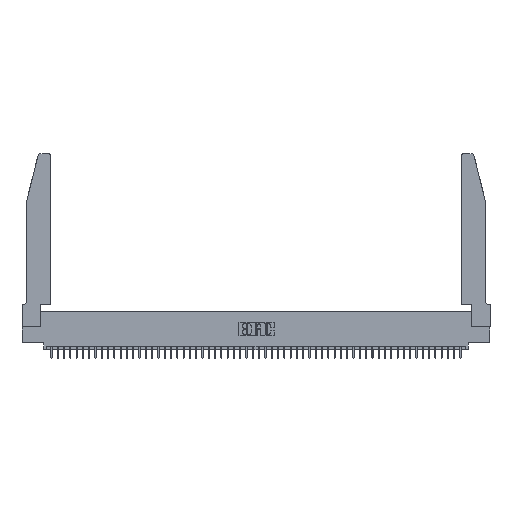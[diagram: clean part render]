
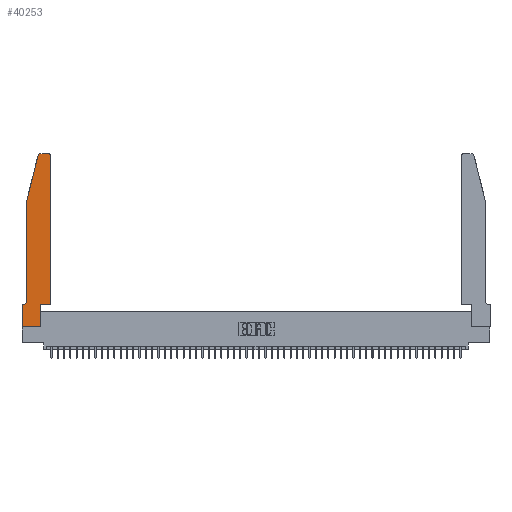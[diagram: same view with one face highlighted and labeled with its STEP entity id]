
A CAD part, top view. The second image highlights one B-rep face of the part: STEP entity #40253.
In plain terms, the highlighted planar face has unit normal (0, 0, 1).
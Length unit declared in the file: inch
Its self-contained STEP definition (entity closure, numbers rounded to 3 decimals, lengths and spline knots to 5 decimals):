
#1168 = CARTESIAN_POINT ( 'NONE',  ( 0.4505, 0.35, 0.37 ) ) ;
#1731 = LINE ( 'NONE', #50038, #8873 ) ;
#2999 = ORIENTED_EDGE ( 'NONE', *, *, #24528, .T. ) ;
#3394 = LINE ( 'NONE', #49758, #8717 ) ;
#3567 = DIRECTION ( 'NONE',  ( -0.239, -0.971, 0. ) ) ;
#3922 = VECTOR ( 'NONE', #53057, 39.37008 ) ;
#4249 = CARTESIAN_POINT ( 'NONE',  ( 0.0055, 0.35, 0.37 ) ) ;
#4438 = CARTESIAN_POINT ( 'NONE',  ( 0.0755, 0.35, 0.37 ) ) ;
#4554 = ORIENTED_EDGE ( 'NONE', *, *, #28800, .T. ) ;
#4902 = CARTESIAN_POINT ( 'NONE',  ( 0.2865, 0.35, 0.37 ) ) ;
#5096 = VECTOR ( 'NONE', #22157, 39.37008 ) ;
#5981 = ORIENTED_EDGE ( 'NONE', *, *, #35964, .T. ) ;
#6367 = ORIENTED_EDGE ( 'NONE', *, *, #37908, .T. ) ;
#6653 = DIRECTION ( 'NONE',  ( 0., -1., 0. ) ) ;
#7056 = CARTESIAN_POINT ( 'NONE',  ( 0.284, 2.75, 0.37 ) ) ;
#7441 = LINE ( 'NONE', #32641, #24389 ) ;
#7539 = CARTESIAN_POINT ( 'NONE',  ( 0.4505, 0.35, 0.37 ) ) ;
#7691 = DIRECTION ( 'NONE',  ( 1., 0., 0. ) ) ;
#7770 = ORIENTED_EDGE ( 'NONE', *, *, #14251, .T. ) ;
#8327 = DIRECTION ( 'NONE',  ( 0., 1., 0. ) ) ;
#8717 = VECTOR ( 'NONE', #20447, 39.37008 ) ;
#8873 = VECTOR ( 'NONE', #37860, 39.37008 ) ;
#9023 = LINE ( 'NONE', #4438, #3922 ) ;
#9691 = LINE ( 'NONE', #26239, #5096 ) ;
#9996 = CIRCLE ( 'NONE', #29907, 0.03 ) ;
#11538 = CARTESIAN_POINT ( 'NONE',  ( 0.4205, 2.72, 0.37 ) ) ;
#12077 = DIRECTION ( 'NONE',  ( 1., 0., 0. ) ) ;
#12919 = ORIENTED_EDGE ( 'NONE', *, *, #52742, .T. ) ;
#13733 = PLANE ( 'NONE',  #42702 ) ;
#13891 = ORIENTED_EDGE ( 'NONE', *, *, #16941, .T. ) ;
#14251 = EDGE_CURVE ( 'NONE', #24270, #21484, #44726, .T. ) ;
#14649 = DIRECTION ( 'NONE',  ( -1., 0., 0. ) ) ;
#16587 = CARTESIAN_POINT ( 'NONE',  ( 0.2865, 0., 0.37 ) ) ;
#16941 = EDGE_CURVE ( 'NONE', #29308, #30890, #9691, .T. ) ;
#19548 = CARTESIAN_POINT ( 'NONE',  ( 0.0755, 2., 0.37 ) ) ;
#19791 = VECTOR ( 'NONE', #32845, 39.37008 ) ;
#20447 = DIRECTION ( 'NONE',  ( 0., -1., 0. ) ) ;
#20902 = ORIENTED_EDGE ( 'NONE', *, *, #30260, .T. ) ;
#21484 = VERTEX_POINT ( 'NONE', #38367 ) ;
#22006 = DIRECTION ( 'NONE',  ( 1., 0., 0. ) ) ;
#22157 = DIRECTION ( 'NONE',  ( 0., 1., 0. ) ) ;
#22595 = CARTESIAN_POINT ( 'NONE',  ( 0.0755, 0.42, 0.37 ) ) ;
#22673 = DIRECTION ( 'NONE',  ( 0., 0., 1. ) ) ;
#22874 = CIRCLE ( 'NONE', #46230, 0.03 ) ;
#23353 = CARTESIAN_POINT ( 'NONE',  ( 0., 0.35, 0.37 ) ) ;
#23642 = LINE ( 'NONE', #19548, #27076 ) ;
#24270 = VERTEX_POINT ( 'NONE', #1168 ) ;
#24389 = VECTOR ( 'NONE', #7691, 39.37008 ) ;
#24528 = EDGE_CURVE ( 'NONE', #47407, #33727, #36673, .T. ) ;
#26138 = EDGE_CURVE ( 'NONE', #39356, #31213, #49394, .T. ) ;
#26239 = CARTESIAN_POINT ( 'NONE',  ( 0.2865, 0.35, 0.37 ) ) ;
#27076 = VECTOR ( 'NONE', #3567, 39.37008 ) ;
#28777 = CARTESIAN_POINT ( 'NONE',  ( 0.2605, 2.75, 0.37 ) ) ;
#28800 = EDGE_CURVE ( 'NONE', #38100, #39356, #3394, .T. ) ;
#29308 = VERTEX_POINT ( 'NONE', #16587 ) ;
#29907 = AXIS2_PLACEMENT_3D ( 'NONE', #11538, #45198, #12077 ) ;
#30260 = EDGE_CURVE ( 'NONE', #30890, #24270, #1731, .T. ) ;
#30359 = CARTESIAN_POINT ( 'NONE',  ( 0.25487, 2.72718, 0.37 ) ) ;
#30890 = VERTEX_POINT ( 'NONE', #4902 ) ;
#31034 = VECTOR ( 'NONE', #8327, 39.37008 ) ;
#31213 = VERTEX_POINT ( 'NONE', #4249 ) ;
#32641 = CARTESIAN_POINT ( 'NONE',  ( 0., 0., 0.37 ) ) ;
#32845 = DIRECTION ( 'NONE',  ( -1., 0., 0. ) ) ;
#33727 = VERTEX_POINT ( 'NONE', #7056 ) ;
#34621 = CARTESIAN_POINT ( 'NONE',  ( 0., 0.35, 0.37 ) ) ;
#34632 = EDGE_CURVE ( 'NONE', #51278, #43472, #43843, .T. ) ;
#35040 = CARTESIAN_POINT ( 'NONE',  ( 0.284, 2.72, 0.37 ) ) ;
#35964 = EDGE_CURVE ( 'NONE', #21484, #47407, #9996, .T. ) ;
#36211 = ORIENTED_EDGE ( 'NONE', *, *, #34632, .T. ) ;
#36673 = LINE ( 'NONE', #28777, #19791 ) ;
#37408 = ORIENTED_EDGE ( 'NONE', *, *, #26138, .T. ) ;
#37506 = EDGE_CURVE ( 'NONE', #43472, #29308, #7441, .T. ) ;
#37860 = DIRECTION ( 'NONE',  ( 1., 0., 0. ) ) ;
#37908 = EDGE_CURVE ( 'NONE', #42637, #38100, #23642, .T. ) ;
#38100 = VERTEX_POINT ( 'NONE', #46133 ) ;
#38367 = CARTESIAN_POINT ( 'NONE',  ( 0.4505, 2.72, 0.37 ) ) ;
#39260 = CARTESIAN_POINT ( 'NONE',  ( 0., 0., 0.37 ) ) ;
#39356 = VERTEX_POINT ( 'NONE', #22595 ) ;
#40253 = ADVANCED_FACE ( 'NONE', ( #43845 ), #13733, .T. ) ;
#42199 = EDGE_CURVE ( 'NONE', #33727, #42637, #22874, .T. ) ;
#42397 = DIRECTION ( 'NONE',  ( 0., 0., 1. ) ) ;
#42637 = VERTEX_POINT ( 'NONE', #30359 ) ;
#42702 = AXIS2_PLACEMENT_3D ( 'NONE', #34621, #22673, #50895 ) ;
#43472 = VERTEX_POINT ( 'NONE', #44634 ) ;
#43843 = LINE ( 'NONE', #39260, #52476 ) ;
#43845 = FACE_OUTER_BOUND ( 'NONE', #44596, .T. ) ;
#44236 = DIRECTION ( 'NONE',  ( 0., 0., -1. ) ) ;
#44503 = CARTESIAN_POINT ( 'NONE',  ( 0.0055, 0.42, 0.37 ) ) ;
#44596 = EDGE_LOOP ( 'NONE', ( #2999, #46722, #6367, #4554, #37408, #12919, #36211, #45774, #13891, #20902, #7770, #5981 ) ) ;
#44634 = CARTESIAN_POINT ( 'NONE',  ( 0., 0., 0.37 ) ) ;
#44726 = LINE ( 'NONE', #7539, #31034 ) ;
#45198 = DIRECTION ( 'NONE',  ( 0., 0., 1. ) ) ;
#45774 = ORIENTED_EDGE ( 'NONE', *, *, #37506, .T. ) ;
#46133 = CARTESIAN_POINT ( 'NONE',  ( 0.0755, 2., 0.37 ) ) ;
#46230 = AXIS2_PLACEMENT_3D ( 'NONE', #35040, #42397, #22006 ) ;
#46722 = ORIENTED_EDGE ( 'NONE', *, *, #42199, .T. ) ;
#47407 = VERTEX_POINT ( 'NONE', #50116 ) ;
#49394 = CIRCLE ( 'NONE', #51973, 0.07 ) ;
#49758 = CARTESIAN_POINT ( 'NONE',  ( 0.0755, 2., 0.37 ) ) ;
#50038 = CARTESIAN_POINT ( 'NONE',  ( 0.4505, 0.35, 0.37 ) ) ;
#50116 = CARTESIAN_POINT ( 'NONE',  ( 0.4205, 2.75, 0.37 ) ) ;
#50895 = DIRECTION ( 'NONE',  ( 1., 0., 0. ) ) ;
#51278 = VERTEX_POINT ( 'NONE', #23353 ) ;
#51973 = AXIS2_PLACEMENT_3D ( 'NONE', #44503, #44236, #14649 ) ;
#52476 = VECTOR ( 'NONE', #6653, 39.37008 ) ;
#52742 = EDGE_CURVE ( 'NONE', #31213, #51278, #9023, .T. ) ;
#53057 = DIRECTION ( 'NONE',  ( -1., 0., 0. ) ) ;
